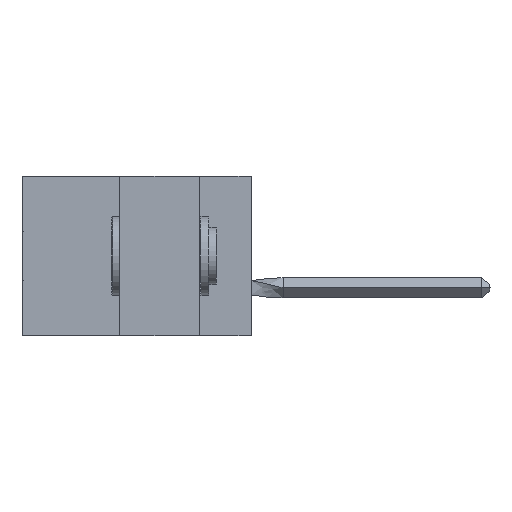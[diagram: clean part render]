
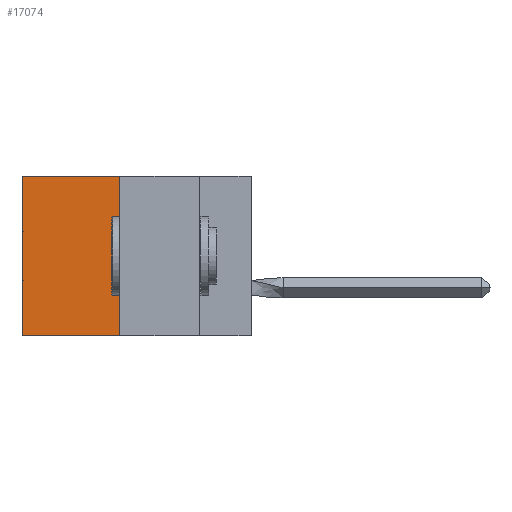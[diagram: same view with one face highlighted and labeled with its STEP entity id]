
A CAD part, left-side view. The second image highlights one B-rep face of the part: STEP entity #17074.
In plain terms, the highlighted planar face has unit normal (-1, 0, 0).
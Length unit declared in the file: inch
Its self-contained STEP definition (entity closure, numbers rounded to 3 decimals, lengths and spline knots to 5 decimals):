
#879 = VERTEX_POINT ( 'NONE', #17540 ) ;
#1223 = EDGE_CURVE ( 'NONE', #12443, #879, #40950, .T. ) ;
#1859 = VECTOR ( 'NONE', #27498, 39.37008 ) ;
#2823 = CARTESIAN_POINT ( 'NONE',  ( 0.305, 0.72, 0. ) ) ;
#3948 = VECTOR ( 'NONE', #4453, 39.37008 ) ;
#4453 = DIRECTION ( 'NONE',  ( 0., 1., 0. ) ) ;
#5382 = VECTOR ( 'NONE', #13835, 39.37008 ) ;
#6046 = CARTESIAN_POINT ( 'NONE',  ( 0.305, 0.72, -0.5 ) ) ;
#7850 = ORIENTED_EDGE ( 'NONE', *, *, #32820, .F. ) ;
#8358 = PLANE ( 'NONE',  #46063 ) ;
#12443 = VERTEX_POINT ( 'NONE', #45881 ) ;
#13420 = LINE ( 'NONE', #44017, #3948 ) ;
#13835 = DIRECTION ( 'NONE',  ( 0., 1., 0. ) ) ;
#16406 = ORIENTED_EDGE ( 'NONE', *, *, #43506, .T. ) ;
#17074 = ADVANCED_FACE ( 'NONE', ( #34509 ), #8358, .F. ) ;
#17540 = CARTESIAN_POINT ( 'NONE',  ( 0.305, 0.413, -0.5 ) ) ;
#20517 = ORIENTED_EDGE ( 'NONE', *, *, #45455, .T. ) ;
#22328 = DIRECTION ( 'NONE',  ( 0., 0., -1. ) ) ;
#23622 = CARTESIAN_POINT ( 'NONE',  ( 0.305, 0.72, -0.5 ) ) ;
#24726 = CARTESIAN_POINT ( 'NONE',  ( 0.305, 0.413, -0.5 ) ) ;
#27123 = LINE ( 'NONE', #24726, #5382 ) ;
#27498 = DIRECTION ( 'NONE',  ( 0., 0., -1. ) ) ;
#29712 = VECTOR ( 'NONE', #22328, 39.37008 ) ;
#32820 = EDGE_CURVE ( 'NONE', #879, #45228, #27123, .T. ) ;
#33259 = DIRECTION ( 'NONE',  ( 0., 0., -1. ) ) ;
#34509 = FACE_OUTER_BOUND ( 'NONE', #37341, .T. ) ;
#36443 = CARTESIAN_POINT ( 'NONE',  ( 0.305, 0.413, -0.5 ) ) ;
#36851 = DIRECTION ( 'NONE',  ( 1., 0., 0. ) ) ;
#37341 = EDGE_LOOP ( 'NONE', ( #20517, #7850, #42893, #16406 ) ) ;
#39626 = VERTEX_POINT ( 'NONE', #2823 ) ;
#40950 = LINE ( 'NONE', #36443, #29712 ) ;
#42893 = ORIENTED_EDGE ( 'NONE', *, *, #1223, .F. ) ;
#43153 = LINE ( 'NONE', #6046, #1859 ) ;
#43506 = EDGE_CURVE ( 'NONE', #12443, #39626, #13420, .T. ) ;
#44017 = CARTESIAN_POINT ( 'NONE',  ( 0.305, 0.413, 0. ) ) ;
#44536 = CARTESIAN_POINT ( 'NONE',  ( 0.305, 0.413, -0.5 ) ) ;
#45228 = VERTEX_POINT ( 'NONE', #23622 ) ;
#45455 = EDGE_CURVE ( 'NONE', #39626, #45228, #43153, .T. ) ;
#45881 = CARTESIAN_POINT ( 'NONE',  ( 0.305, 0.413, 0. ) ) ;
#46063 = AXIS2_PLACEMENT_3D ( 'NONE', #44536, #36851, #33259 ) ;
